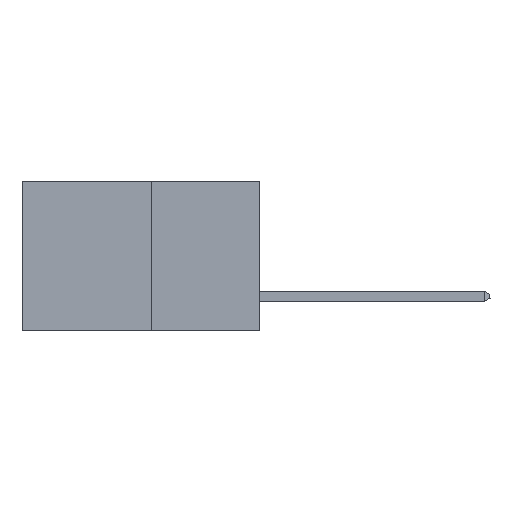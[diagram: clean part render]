
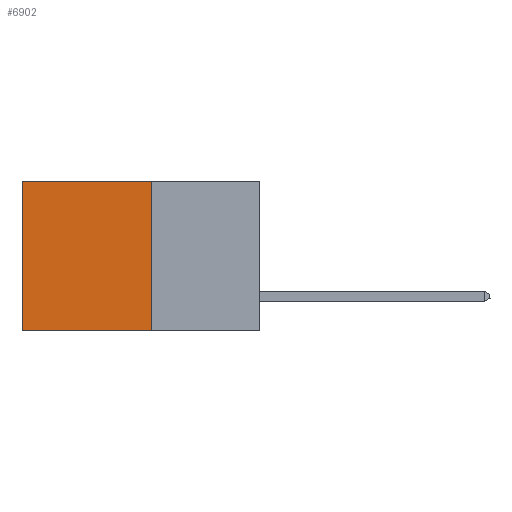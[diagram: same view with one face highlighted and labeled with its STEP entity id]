
A CAD part, left-side view. The second image highlights one B-rep face of the part: STEP entity #6902.
In plain terms, the highlighted planar face has unit normal (-1, 0, 0).
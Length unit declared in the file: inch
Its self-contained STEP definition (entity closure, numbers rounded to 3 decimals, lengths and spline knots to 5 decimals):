
#1027 = CARTESIAN_POINT ( 'NONE',  ( 0.277, 0.27, -0.37 ) ) ;
#2280 = CARTESIAN_POINT ( 'NONE',  ( 0.277, 0.27, 0. ) ) ;
#2864 = ORIENTED_EDGE ( 'NONE', *, *, #7593, .F. ) ;
#3686 = DIRECTION ( 'NONE',  ( 0., 0., -1. ) ) ;
#4111 = EDGE_LOOP ( 'NONE', ( #13460, #20389, #2864, #19775 ) ) ;
#4412 = VERTEX_POINT ( 'NONE', #1027 ) ;
#4523 = VECTOR ( 'NONE', #5354, 39.37008 ) ;
#4761 = DIRECTION ( 'NONE',  ( 0., 0., -1. ) ) ;
#5304 = VECTOR ( 'NONE', #21319, 39.37008 ) ;
#5354 = DIRECTION ( 'NONE',  ( 0., 0., -1. ) ) ;
#6112 = LINE ( 'NONE', #2280, #19634 ) ;
#6902 = ADVANCED_FACE ( 'NONE', ( #12660 ), #23843, .F. ) ;
#7593 = EDGE_CURVE ( 'NONE', #21468, #4412, #23492, .T. ) ;
#9890 = VERTEX_POINT ( 'NONE', #14657 ) ;
#12242 = CARTESIAN_POINT ( 'NONE',  ( 0.277, 0.27, -0.37 ) ) ;
#12660 = FACE_OUTER_BOUND ( 'NONE', #4111, .T. ) ;
#13221 = EDGE_CURVE ( 'NONE', #17040, #9890, #14515, .T. ) ;
#13387 = DIRECTION ( 'NONE',  ( 0., 1., 0. ) ) ;
#13460 = ORIENTED_EDGE ( 'NONE', *, *, #13221, .T. ) ;
#14515 = LINE ( 'NONE', #21263, #23625 ) ;
#14657 = CARTESIAN_POINT ( 'NONE',  ( 0.277, 0.59, -0.37 ) ) ;
#14775 = DIRECTION ( 'NONE',  ( 1., 0., 0. ) ) ;
#15160 = LINE ( 'NONE', #12242, #5304 ) ;
#17040 = VERTEX_POINT ( 'NONE', #23691 ) ;
#18269 = CARTESIAN_POINT ( 'NONE',  ( 0.277, 0.27, -0.37 ) ) ;
#18877 = AXIS2_PLACEMENT_3D ( 'NONE', #22041, #14775, #3686 ) ;
#19197 = CARTESIAN_POINT ( 'NONE',  ( 0.277, 0.27, 0. ) ) ;
#19363 = EDGE_CURVE ( 'NONE', #4412, #9890, #15160, .T. ) ;
#19634 = VECTOR ( 'NONE', #13387, 39.37008 ) ;
#19775 = ORIENTED_EDGE ( 'NONE', *, *, #20861, .T. ) ;
#20389 = ORIENTED_EDGE ( 'NONE', *, *, #19363, .F. ) ;
#20861 = EDGE_CURVE ( 'NONE', #21468, #17040, #6112, .T. ) ;
#21263 = CARTESIAN_POINT ( 'NONE',  ( 0.277, 0.59, -0.37 ) ) ;
#21319 = DIRECTION ( 'NONE',  ( 0., 1., 0. ) ) ;
#21468 = VERTEX_POINT ( 'NONE', #19197 ) ;
#22041 = CARTESIAN_POINT ( 'NONE',  ( 0.277, 0.27, -0.37 ) ) ;
#23492 = LINE ( 'NONE', #18269, #4523 ) ;
#23625 = VECTOR ( 'NONE', #4761, 39.37008 ) ;
#23691 = CARTESIAN_POINT ( 'NONE',  ( 0.277, 0.59, 0. ) ) ;
#23843 = PLANE ( 'NONE',  #18877 ) ;
